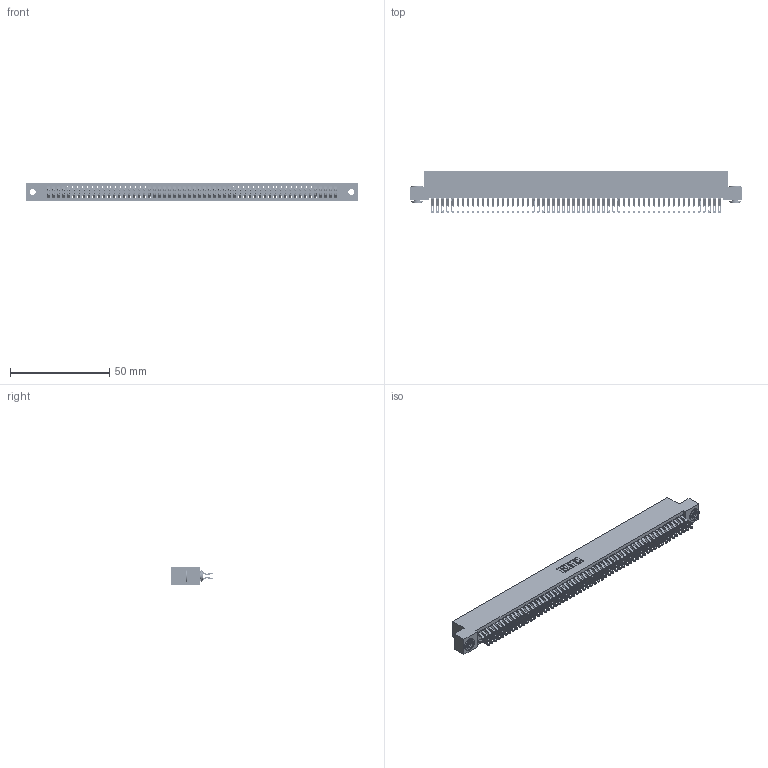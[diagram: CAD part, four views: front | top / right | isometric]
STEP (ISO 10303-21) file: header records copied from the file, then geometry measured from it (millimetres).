
FILE_DESCRIPTION (( 'STEP AP203' ), '1' );
FILE_NAME ('342-116-555-203.STEP', '2018-08-14T13:49:44', ( '' ), ( '' ), 'SwSTEP 2.0', 'SolidWorks 2016', '' );
FILE_SCHEMA (( 'CONFIG_CONTROL_DESIGN' ));
Length unit declared in the file: inch
Products named in the file (4): 342-116-555-203; 342 Part_.156 TH; 342-250-002_345-250-002-102; 345-292-001_555 Tail
Assembly tree (119 placements, depth 2):
  342-116-555-203
    342 Part_.156 TH
    345-292-001_555 Tail  x116
    342-250-002_345-250-002-102  x2
Bounding box: 167.64 x 21.47 x 9.4 mm (x, y, z)
Volume: 15483.3 mm3; surface area: 26933.7 mm2
Topology: 119 solids, 119 shells, 6876 faces, 21603 edges, 14398 vertices
Faces by surface type: plane 4020, cylinder 2848, cone 8
Entity records: 36088 total; most frequent: CARTESIAN_POINT 5971, ORIENTED_EDGE 5870, DIRECTION 5077, EDGE_CURVE 2935, VECTOR 2763, LINE 2763, VERTEX_POINT 1954, AXIS2_PLACEMENT_3D 1157
